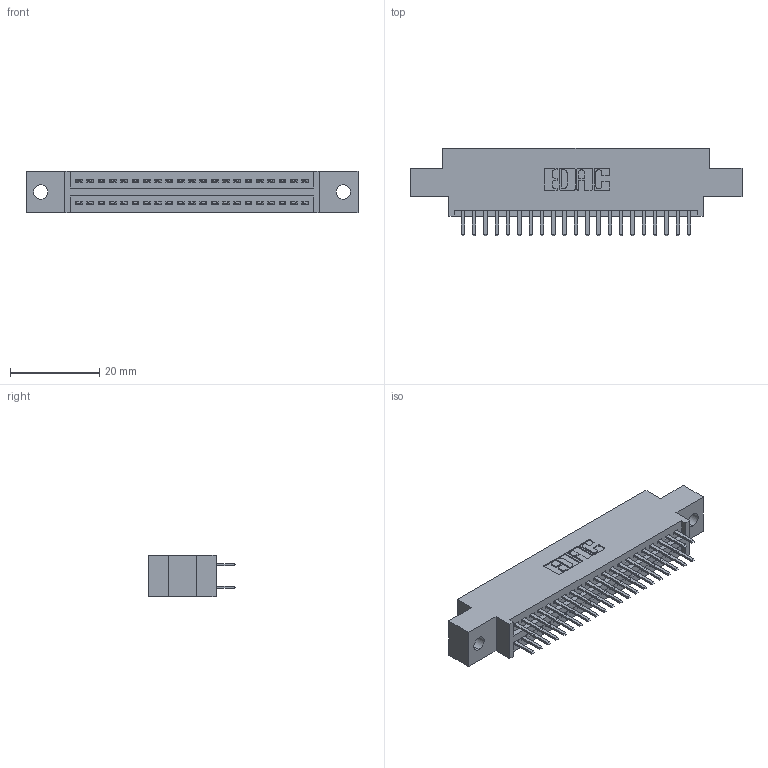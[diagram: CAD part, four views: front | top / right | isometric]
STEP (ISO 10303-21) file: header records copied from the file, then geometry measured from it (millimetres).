
FILE_DESCRIPTION (( 'STEP AP203' ), '1' );
FILE_NAME ('395-042-520-802.STEP', '2018-11-15T07:43:41', ( '' ), ( '' ), 'SwSTEP 2.0', 'SolidWorks 2016', '' );
FILE_SCHEMA (( 'CONFIG_CONTROL_DESIGN' ));
Length unit declared in the file: inch
Products named in the file (3): 345 Part_0.170 Offset - 0.128 Dia; 345-292-001_345-293-120; 395-042-520-802
Assembly tree (43 placements, depth 2):
  395-042-520-802
    345 Part_0.170 Offset - 0.128 Dia
    345-292-001_345-293-120  x42
Bounding box: 74.55 x 19.68 x 9.4 mm (x, y, z)
Volume: 6878.3 mm3; surface area: 9592 mm2
Topology: 43 solids, 43 shells, 2398 faces, 6947 edges, 4518 vertices
Faces by surface type: plane 1554, cylinder 844
Entity records: 19553 total; most frequent: CARTESIAN_POINT 3312, ORIENTED_EDGE 3234, DIRECTION 2933, EDGE_CURVE 1617, VECTOR 1397, LINE 1397, VERTEX_POINT 1074, AXIS2_PLACEMENT_3D 768
